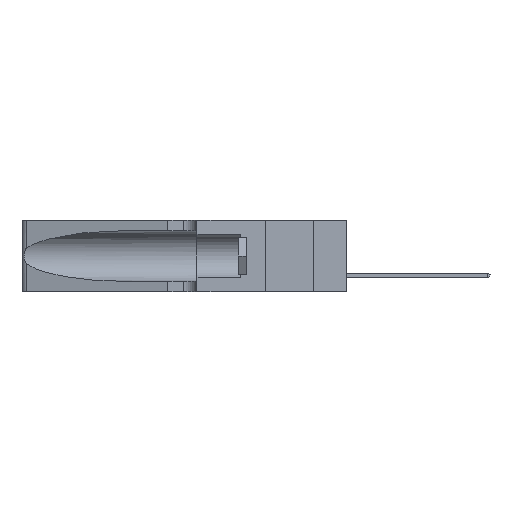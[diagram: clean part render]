
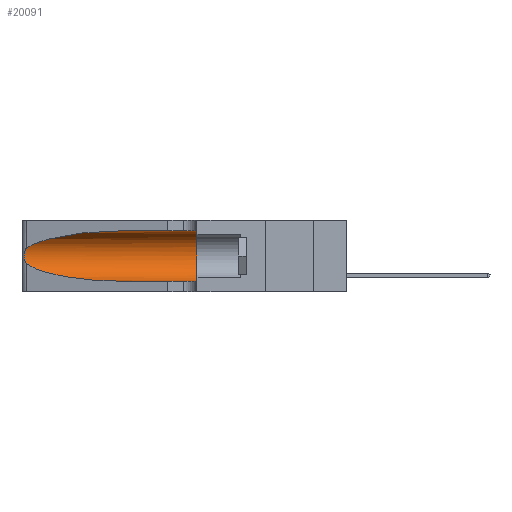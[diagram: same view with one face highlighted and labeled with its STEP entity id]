
A CAD part, left-side view. The second image highlights one B-rep face of the part: STEP entity #20091.
In plain terms, the highlighted cylindrical face has radius 3.308 mm (diameter 6.617 mm), a partial arc.
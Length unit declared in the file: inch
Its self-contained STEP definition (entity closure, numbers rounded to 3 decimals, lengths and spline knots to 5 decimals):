
#1238 = AXIS2_PLACEMENT_3D ( 'NONE', #17086, #8067, #3984 ) ;
#1555 = CARTESIAN_POINT ( 'NONE',  ( 0.1305, 0.72297, 0.31525 ) ) ;
#3804 = EDGE_CURVE ( 'NONE', #11947, #11354, #11638, .T. ) ;
#3840 = CARTESIAN_POINT ( 'NONE',  ( 0.25487, 1.22718, 0.14631 ) ) ;
#3971 = FACE_OUTER_BOUND ( 'NONE', #20441, .T. ) ;
#3984 = DIRECTION ( 'NONE',  ( 0., 0., -1. ) ) ;
#4528 = VECTOR ( 'NONE', #19801, 39.37008 ) ;
#4688 = CARTESIAN_POINT ( 'NONE',  ( 0.1305, 0.35, 0.05475 ) ) ;
#5215 = LINE ( 'NONE', #24166, #4528 ) ;
#5442 = EDGE_CURVE ( 'NONE', #24048, #19891, #5215, .T. ) ;
#5633 = ORIENTED_EDGE ( 'NONE', *, *, #20419, .T. ) ;
#6606 = CARTESIAN_POINT ( 'NONE',  ( 0.25487, 1.22718, 0.22369 ) ) ;
#7025 = CYLINDRICAL_SURFACE ( 'NONE', #1238, 0.13025 ) ;
#7709 = DIRECTION ( 'NONE',  ( 0., -1., 0. ) ) ;
#8067 = DIRECTION ( 'NONE',  ( 0., -1., 0. ) ) ;
#8668 = CARTESIAN_POINT ( 'NONE',  ( 0.25487, 1.22718, 0.22369 ) ) ;
#10467 = VERTEX_POINT ( 'NONE', #4688 ) ;
#10618 = CARTESIAN_POINT ( 'NONE',  ( 0.25639, 1.23186, 0.15144 ) ) ;
#10804 = CARTESIAN_POINT ( 'NONE',  ( 0.26075, 1.23896, 0.19203 ) ) ;
#10835 = CARTESIAN_POINT ( 'NONE',  ( 0.18966, 0.96281, 0.31525 ) ) ;
#11133 = B_SPLINE_CURVE_WITH_KNOTS ( 'NONE', 3,
 ( #8668, #23777, #12993, #27859, #17017, #12704, #10804, #26011, #21444, #21544, #25805, #10618, #12796, #28053 ),
 .UNSPECIFIED., .F., .F.,
 ( 4, 2, 2, 2, 2, 2, 4 ),
 ( 0., 0.00027, 0.00053, 0.00107, 0.0016, 0.00187, 0.00214 ),
 .UNSPECIFIED. ) ;
#11184 = EDGE_CURVE ( 'NONE', #24048, #23689, #16225, .T. ) ;
#11354 = VERTEX_POINT ( 'NONE', #11819 ) ;
#11638 =( BOUNDED_CURVE ( )  B_SPLINE_CURVE ( 3, ( #15104, #19193, #21435, #25698 ),
 .UNSPECIFIED., .F., .F. ) 
 B_SPLINE_CURVE_WITH_KNOTS ( ( 4, 4 ),
 ( 3.44316, 4.71239 ),
 .UNSPECIFIED. ) 
 CURVE ( )  GEOMETRIC_REPRESENTATION_ITEM ( )  RATIONAL_B_SPLINE_CURVE ( ( 1., 0.87, 0.87, 1. ) ) 
 REPRESENTATION_ITEM ( '' )  );
#11819 = CARTESIAN_POINT ( 'NONE',  ( 0.1305, 0.72297, 0.05475 ) ) ;
#11840 = CARTESIAN_POINT ( 'NONE',  ( 0.1305, 1.61858, 0.05475 ) ) ;
#11947 = VERTEX_POINT ( 'NONE', #3840 ) ;
#12357 = CIRCLE ( 'NONE', #16847, 0.13025 ) ;
#12704 = CARTESIAN_POINT ( 'NONE',  ( 0.26018, 1.23835, 0.19895 ) ) ;
#12796 = CARTESIAN_POINT ( 'NONE',  ( 0.25555, 1.22993, 0.14849 ) ) ;
#12993 = CARTESIAN_POINT ( 'NONE',  ( 0.25639, 1.23184, 0.21858 ) ) ;
#13371 = EDGE_CURVE ( 'NONE', #23689, #11947, #11133, .T. ) ;
#15104 = CARTESIAN_POINT ( 'NONE',  ( 0.25487, 1.22718, 0.14631 ) ) ;
#15833 = LINE ( 'NONE', #11840, #26341 ) ;
#16225 =( BOUNDED_CURVE ( )  B_SPLINE_CURVE ( 3, ( #19435, #10835, #17432, #6606 ),
 .UNSPECIFIED., .F., .F. ) 
 B_SPLINE_CURVE_WITH_KNOTS ( ( 4, 4 ),
 ( 1.5708, 2.84003 ),
 .UNSPECIFIED. ) 
 CURVE ( )  GEOMETRIC_REPRESENTATION_ITEM ( )  RATIONAL_B_SPLINE_CURVE ( ( 1., 0.87, 0.87, 1. ) ) 
 REPRESENTATION_ITEM ( '' )  );
#16847 = AXIS2_PLACEMENT_3D ( 'NONE', #25233, #25039, #18451 ) ;
#17017 = CARTESIAN_POINT ( 'NONE',  ( 0.25854, 1.2359, 0.20912 ) ) ;
#17086 = CARTESIAN_POINT ( 'NONE',  ( 0.1305, 1.61858, 0.185 ) ) ;
#17432 = CARTESIAN_POINT ( 'NONE',  ( 0.2373, 1.15595, 0.28018 ) ) ;
#17626 = ORIENTED_EDGE ( 'NONE', *, *, #5442, .F. ) ;
#17845 = ORIENTED_EDGE ( 'NONE', *, *, #13371, .T. ) ;
#18310 = ORIENTED_EDGE ( 'NONE', *, *, #27658, .F. ) ;
#18451 = DIRECTION ( 'NONE',  ( 0., 0., 1. ) ) ;
#19193 = CARTESIAN_POINT ( 'NONE',  ( 0.2373, 1.15595, 0.08982 ) ) ;
#19435 = CARTESIAN_POINT ( 'NONE',  ( 0.1305, 0.72297, 0.31525 ) ) ;
#19801 = DIRECTION ( 'NONE',  ( 0., -1., 0. ) ) ;
#19891 = VERTEX_POINT ( 'NONE', #20546 ) ;
#20091 = ADVANCED_FACE ( 'NONE', ( #3971 ), #7025, .F. ) ;
#20419 = EDGE_CURVE ( 'NONE', #11354, #10467, #15833, .T. ) ;
#20441 = EDGE_LOOP ( 'NONE', ( #26964, #17845, #21136, #5633, #18310, #17626 ) ) ;
#20546 = CARTESIAN_POINT ( 'NONE',  ( 0.1305, 0.35, 0.31525 ) ) ;
#21136 = ORIENTED_EDGE ( 'NONE', *, *, #3804, .T. ) ;
#21435 = CARTESIAN_POINT ( 'NONE',  ( 0.18966, 0.96281, 0.05475 ) ) ;
#21444 = CARTESIAN_POINT ( 'NONE',  ( 0.26017, 1.23833, 0.17102 ) ) ;
#21544 = CARTESIAN_POINT ( 'NONE',  ( 0.25856, 1.23593, 0.16098 ) ) ;
#23689 = VERTEX_POINT ( 'NONE', #25415 ) ;
#23777 = CARTESIAN_POINT ( 'NONE',  ( 0.25555, 1.22994, 0.2215 ) ) ;
#24048 = VERTEX_POINT ( 'NONE', #1555 ) ;
#24166 = CARTESIAN_POINT ( 'NONE',  ( 0.1305, 1.61858, 0.31525 ) ) ;
#25039 = DIRECTION ( 'NONE',  ( 0., 1., 0. ) ) ;
#25233 = CARTESIAN_POINT ( 'NONE',  ( 0.1305, 0.35, 0.185 ) ) ;
#25415 = CARTESIAN_POINT ( 'NONE',  ( 0.25487, 1.22718, 0.22369 ) ) ;
#25698 = CARTESIAN_POINT ( 'NONE',  ( 0.1305, 0.72297, 0.05475 ) ) ;
#25805 = CARTESIAN_POINT ( 'NONE',  ( 0.25789, 1.23486, 0.15765 ) ) ;
#26011 = CARTESIAN_POINT ( 'NONE',  ( 0.26075, 1.23896, 0.178 ) ) ;
#26341 = VECTOR ( 'NONE', #7709, 39.37008 ) ;
#26964 = ORIENTED_EDGE ( 'NONE', *, *, #11184, .T. ) ;
#27658 = EDGE_CURVE ( 'NONE', #19891, #10467, #12357, .T. ) ;
#27859 = CARTESIAN_POINT ( 'NONE',  ( 0.25787, 1.23484, 0.2124 ) ) ;
#28053 = CARTESIAN_POINT ( 'NONE',  ( 0.25487, 1.22718, 0.14631 ) ) ;
